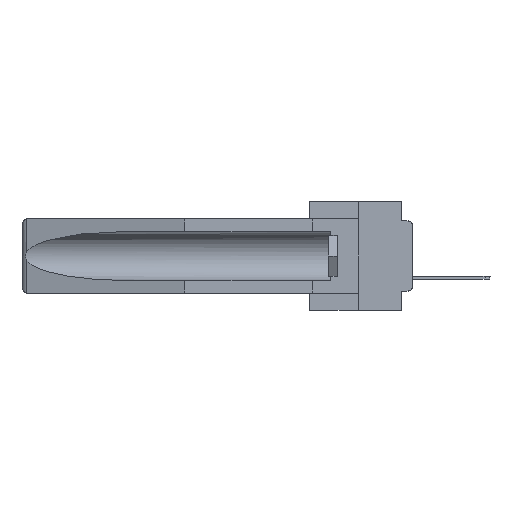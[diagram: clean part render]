
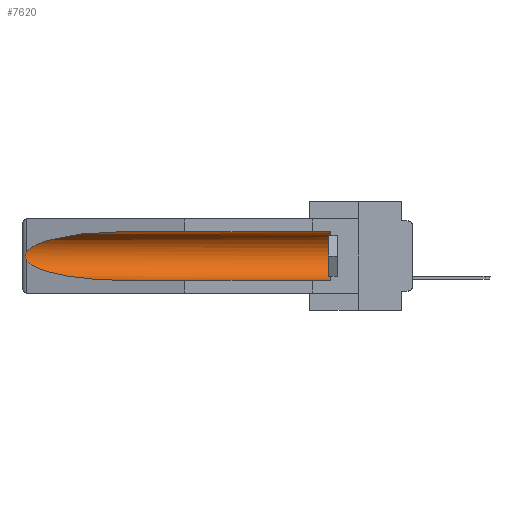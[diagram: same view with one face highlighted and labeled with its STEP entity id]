
A CAD part, left-side view. The second image highlights one B-rep face of the part: STEP entity #7620.
In plain terms, the highlighted cylindrical face has radius 2.857 mm (diameter 5.715 mm), a partial arc.
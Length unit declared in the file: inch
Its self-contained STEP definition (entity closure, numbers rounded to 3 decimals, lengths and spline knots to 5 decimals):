
#478 = CARTESIAN_POINT ( 'NONE',  ( 0.155, 1.07973, -0.284 ) ) ;
#760 =( BOUNDED_CURVE ( )  B_SPLINE_CURVE ( 3, ( #5539, #27035, #3472, #20621 ),
 .UNSPECIFIED., .F., .F. ) 
 B_SPLINE_CURVE_WITH_KNOTS ( ( 4, 4 ),
 ( 4.71239, 6.08839 ),
 .UNSPECIFIED. ) 
 CURVE ( )  GEOMETRIC_REPRESENTATION_ITEM ( )  RATIONAL_B_SPLINE_CURVE ( ( 1., 0.848, 0.848, 1. ) ) 
 REPRESENTATION_ITEM ( '' )  );
#1663 = VERTEX_POINT ( 'NONE', #20391 ) ;
#2581 = CARTESIAN_POINT ( 'NONE',  ( 0.26537, 1.52718, -0.19328 ) ) ;
#3143 = DIRECTION ( 'NONE',  ( 0., 1., 0. ) ) ;
#3472 = CARTESIAN_POINT ( 'NONE',  ( 0.25451, 1.48313, -0.09465 ) ) ;
#4618 = CARTESIAN_POINT ( 'NONE',  ( 0.26537, 1.52718, -0.19328 ) ) ;
#5221 = VERTEX_POINT ( 'NONE', #27431 ) ;
#5539 = CARTESIAN_POINT ( 'NONE',  ( 0.155, 1.07973, -0.059 ) ) ;
#5543 = FACE_OUTER_BOUND ( 'NONE', #16665, .T. ) ;
#6686 = VERTEX_POINT ( 'NONE', #8446 ) ;
#7226 = VECTOR ( 'NONE', #25919, 39.37008 ) ;
#7443 = CIRCLE ( 'NONE', #21081, 0.1125 ) ;
#7620 = ADVANCED_FACE ( 'NONE', ( #5543 ), #26309, .F. ) ;
#8196 = ORIENTED_EDGE ( 'NONE', *, *, #19199, .T. ) ;
#8352 = ORIENTED_EDGE ( 'NONE', *, *, #25827, .T. ) ;
#8357 = CARTESIAN_POINT ( 'NONE',  ( 0.26537, 1.52718, -0.14972 ) ) ;
#8383 = CARTESIAN_POINT ( 'NONE',  ( 0.26654, 1.53092, -0.15636 ) ) ;
#8446 = CARTESIAN_POINT ( 'NONE',  ( 0.155, 0.126, -0.059 ) ) ;
#8727 = CARTESIAN_POINT ( 'NONE',  ( 0.155, -0.30754, -0.059 ) ) ;
#9262 = CARTESIAN_POINT ( 'NONE',  ( 0.26597, 1.5296, -0.19026 ) ) ;
#10377 = VERTEX_POINT ( 'NONE', #4618 ) ;
#11270 = ORIENTED_EDGE ( 'NONE', *, *, #26679, .F. ) ;
#13880 =( BOUNDED_CURVE ( )  B_SPLINE_CURVE ( 3, ( #2581, #17831, #24058, #478 ),
 .UNSPECIFIED., .F., .F. ) 
 B_SPLINE_CURVE_WITH_KNOTS ( ( 4, 4 ),
 ( 0.1948, 1.5708 ),
 .UNSPECIFIED. ) 
 CURVE ( )  GEOMETRIC_REPRESENTATION_ITEM ( )  RATIONAL_B_SPLINE_CURVE ( ( 1., 0.848, 0.848, 1. ) ) 
 REPRESENTATION_ITEM ( '' )  );
#14365 = CARTESIAN_POINT ( 'NONE',  ( 0.155, -0.30754, -0.284 ) ) ;
#14445 = EDGE_CURVE ( 'NONE', #1663, #24788, #760, .T. ) ;
#15592 = CARTESIAN_POINT ( 'NONE',  ( 0.2675, 1.53308, -0.17534 ) ) ;
#16118 = AXIS2_PLACEMENT_3D ( 'NONE', #24157, #16630, #25769 ) ;
#16630 = DIRECTION ( 'NONE',  ( 0., 1., 0. ) ) ;
#16665 = EDGE_LOOP ( 'NONE', ( #19459, #8352, #24069, #11270, #8196, #26538 ) ) ;
#17175 = CARTESIAN_POINT ( 'NONE',  ( 0.2673, 1.5327, -0.16383 ) ) ;
#17642 = CARTESIAN_POINT ( 'NONE',  ( 0.26537, 1.52718, -0.14972 ) ) ;
#17672 = CARTESIAN_POINT ( 'NONE',  ( 0.2673, 1.53269, -0.17917 ) ) ;
#17831 = CARTESIAN_POINT ( 'NONE',  ( 0.25451, 1.48313, -0.24835 ) ) ;
#18730 = CARTESIAN_POINT ( 'NONE',  ( 0.155, 0.126, -0.1715 ) ) ;
#19199 = EDGE_CURVE ( 'NONE', #5221, #6686, #7443, .T. ) ;
#19459 = ORIENTED_EDGE ( 'NONE', *, *, #14445, .T. ) ;
#19535 = LINE ( 'NONE', #8727, #7226 ) ;
#20391 = CARTESIAN_POINT ( 'NONE',  ( 0.155, 1.07973, -0.059 ) ) ;
#20621 = CARTESIAN_POINT ( 'NONE',  ( 0.26537, 1.52718, -0.14972 ) ) ;
#21081 = AXIS2_PLACEMENT_3D ( 'NONE', #18730, #22946, #27396 ) ;
#21335 = CARTESIAN_POINT ( 'NONE',  ( 0.26655, 1.53094, -0.18657 ) ) ;
#22183 = CARTESIAN_POINT ( 'NONE',  ( 0.26537, 1.52718, -0.19328 ) ) ;
#22414 = EDGE_CURVE ( 'NONE', #6686, #1663, #19535, .T. ) ;
#22946 = DIRECTION ( 'NONE',  ( 0., -1., 0. ) ) ;
#23078 = B_SPLINE_CURVE_WITH_KNOTS ( 'NONE', 3,
 ( #8357, #27356, #8383, #17175, #25350, #15592, #17672, #21335, #9262, #22183 ),
 .UNSPECIFIED., .F., .F.,
 ( 4, 2, 2, 2, 4 ),
 ( 0., 0.00029, 0.00058, 0.00087, 0.00117 ),
 .UNSPECIFIED. ) ;
#24058 = CARTESIAN_POINT ( 'NONE',  ( 0.21114, 1.30732, -0.284 ) ) ;
#24069 = ORIENTED_EDGE ( 'NONE', *, *, #24811, .T. ) ;
#24157 = CARTESIAN_POINT ( 'NONE',  ( 0.155, -0.30754, -0.1715 ) ) ;
#24788 = VERTEX_POINT ( 'NONE', #17642 ) ;
#24811 = EDGE_CURVE ( 'NONE', #10377, #26720, #13880, .T. ) ;
#25350 = CARTESIAN_POINT ( 'NONE',  ( 0.2675, 1.53308, -0.16763 ) ) ;
#25716 = LINE ( 'NONE', #14365, #26049 ) ;
#25769 = DIRECTION ( 'NONE',  ( 0., 0., 1. ) ) ;
#25827 = EDGE_CURVE ( 'NONE', #24788, #10377, #23078, .T. ) ;
#25919 = DIRECTION ( 'NONE',  ( 0., 1., 0. ) ) ;
#26049 = VECTOR ( 'NONE', #3143, 39.37008 ) ;
#26309 = CYLINDRICAL_SURFACE ( 'NONE', #16118, 0.1125 ) ;
#26538 = ORIENTED_EDGE ( 'NONE', *, *, #22414, .T. ) ;
#26679 = EDGE_CURVE ( 'NONE', #5221, #26720, #25716, .T. ) ;
#26720 = VERTEX_POINT ( 'NONE', #27344 ) ;
#27035 = CARTESIAN_POINT ( 'NONE',  ( 0.21114, 1.30732, -0.059 ) ) ;
#27344 = CARTESIAN_POINT ( 'NONE',  ( 0.155, 1.07973, -0.284 ) ) ;
#27356 = CARTESIAN_POINT ( 'NONE',  ( 0.26597, 1.52961, -0.15275 ) ) ;
#27396 = DIRECTION ( 'NONE',  ( 0., 0., 1. ) ) ;
#27431 = CARTESIAN_POINT ( 'NONE',  ( 0.155, 0.126, -0.284 ) ) ;
